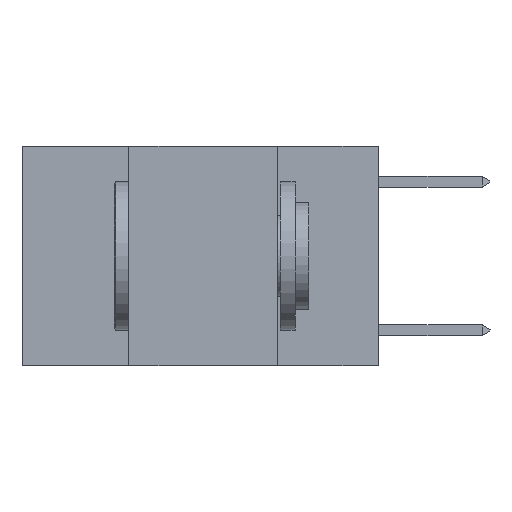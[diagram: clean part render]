
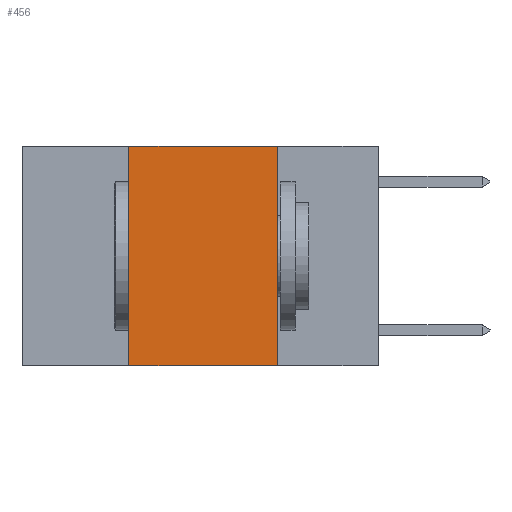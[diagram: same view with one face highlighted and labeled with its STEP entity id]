
A CAD part, left-side view. The second image highlights one B-rep face of the part: STEP entity #456.
In plain terms, the highlighted planar face has unit normal (-1, 0, 0).
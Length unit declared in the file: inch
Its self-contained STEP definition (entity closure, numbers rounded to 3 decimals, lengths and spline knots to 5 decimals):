
#87 = LINE ( 'NONE', #17699, #11779 ) ;
#456 = ADVANCED_FACE ( 'NONE', ( #4935 ), #4644, .F. ) ;
#2348 = VECTOR ( 'NONE', #28603, 39.37008 ) ;
#2505 = LINE ( 'NONE', #26459, #2348 ) ;
#2851 = VERTEX_POINT ( 'NONE', #28571 ) ;
#2936 = LINE ( 'NONE', #9718, #7723 ) ;
#3073 = DIRECTION ( 'NONE',  ( 0., 0., -1. ) ) ;
#3156 = DIRECTION ( 'NONE',  ( 1., 0., 0. ) ) ;
#3753 = VERTEX_POINT ( 'NONE', #15000 ) ;
#4139 = CARTESIAN_POINT ( 'NONE',  ( 0., 0.6, 0. ) ) ;
#4644 = PLANE ( 'NONE',  #11088 ) ;
#4935 = FACE_OUTER_BOUND ( 'NONE', #18290, .T. ) ;
#5221 = CARTESIAN_POINT ( 'NONE',  ( 0., 0.17, 0. ) ) ;
#6113 = ORIENTED_EDGE ( 'NONE', *, *, #27476, .F. ) ;
#7001 = LINE ( 'NONE', #10405, #18481 ) ;
#7370 = ORIENTED_EDGE ( 'NONE', *, *, #22483, .F. ) ;
#7723 = VECTOR ( 'NONE', #12015, 39.37008 ) ;
#9718 = CARTESIAN_POINT ( 'NONE',  ( 0., 0.6, 0. ) ) ;
#9848 = VERTEX_POINT ( 'NONE', #29356 ) ;
#10405 = CARTESIAN_POINT ( 'NONE',  ( 0., 0.17, 0. ) ) ;
#11088 = AXIS2_PLACEMENT_3D ( 'NONE', #4139, #3156, #3073 ) ;
#11443 = VERTEX_POINT ( 'NONE', #5221 ) ;
#11779 = VECTOR ( 'NONE', #19933, 39.37008 ) ;
#12015 = DIRECTION ( 'NONE',  ( 0., -1., 0. ) ) ;
#12670 = DIRECTION ( 'NONE',  ( 0., 0., -1. ) ) ;
#15000 = CARTESIAN_POINT ( 'NONE',  ( 0., 0.17, -0.37 ) ) ;
#15556 = EDGE_CURVE ( 'NONE', #9848, #2851, #2505, .T. ) ;
#17699 = CARTESIAN_POINT ( 'NONE',  ( 0., 0.6, -0.37 ) ) ;
#18290 = EDGE_LOOP ( 'NONE', ( #7370, #6113, #26310, #23787 ) ) ;
#18481 = VECTOR ( 'NONE', #12670, 39.37008 ) ;
#19933 = DIRECTION ( 'NONE',  ( 0., -1., 0. ) ) ;
#21560 = EDGE_CURVE ( 'NONE', #9848, #3753, #87, .T. ) ;
#22483 = EDGE_CURVE ( 'NONE', #11443, #3753, #7001, .T. ) ;
#23787 = ORIENTED_EDGE ( 'NONE', *, *, #21560, .T. ) ;
#26310 = ORIENTED_EDGE ( 'NONE', *, *, #15556, .F. ) ;
#26459 = CARTESIAN_POINT ( 'NONE',  ( 0., 0.42, 0. ) ) ;
#27476 = EDGE_CURVE ( 'NONE', #2851, #11443, #2936, .T. ) ;
#28571 = CARTESIAN_POINT ( 'NONE',  ( 0., 0.42, 0. ) ) ;
#28603 = DIRECTION ( 'NONE',  ( 0., 0., 1. ) ) ;
#29356 = CARTESIAN_POINT ( 'NONE',  ( 0., 0.42, -0.37 ) ) ;
